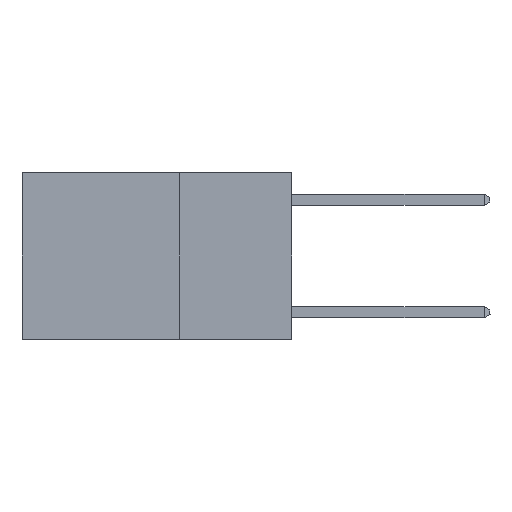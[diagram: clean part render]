
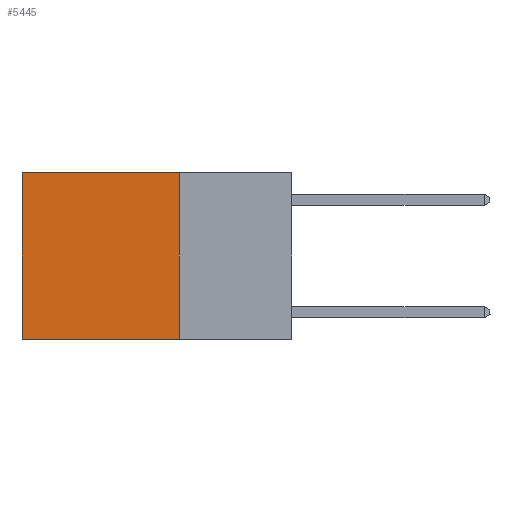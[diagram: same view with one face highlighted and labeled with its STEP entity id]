
A CAD part, left-side view. The second image highlights one B-rep face of the part: STEP entity #5445.
In plain terms, the highlighted planar face has unit normal (-1, 0, 0).
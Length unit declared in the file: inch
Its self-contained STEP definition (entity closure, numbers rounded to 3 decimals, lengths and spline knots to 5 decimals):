
#27 = CARTESIAN_POINT ( 'NONE',  ( 0.2625, 0.6, 0. ) ) ;
#120 = ORIENTED_EDGE ( 'NONE', *, *, #5655, .T. ) ;
#579 = CARTESIAN_POINT ( 'NONE',  ( 0.2625, 0.25, -0.37 ) ) ;
#905 = CARTESIAN_POINT ( 'NONE',  ( 0.2625, 0.6, 0. ) ) ;
#1513 = VECTOR ( 'NONE', #4620, 39.37008 ) ;
#1667 = CARTESIAN_POINT ( 'NONE',  ( 0.2625, 0.25, 0. ) ) ;
#3441 = VECTOR ( 'NONE', #10141, 39.37008 ) ;
#3451 = EDGE_CURVE ( 'NONE', #8773, #9184, #8191, .T. ) ;
#4213 = VERTEX_POINT ( 'NONE', #6761 ) ;
#4579 = EDGE_LOOP ( 'NONE', ( #120, #8152, #8358, #5119 ) ) ;
#4620 = DIRECTION ( 'NONE',  ( 0., 1., 0. ) ) ;
#4699 = AXIS2_PLACEMENT_3D ( 'NONE', #8420, #5802, #8320 ) ;
#4772 = CARTESIAN_POINT ( 'NONE',  ( 0.2625, 0.25, 0. ) ) ;
#4924 = EDGE_CURVE ( 'NONE', #5076, #4213, #8097, .T. ) ;
#5031 = DIRECTION ( 'NONE',  ( 0., 0., -1. ) ) ;
#5076 = VERTEX_POINT ( 'NONE', #579 ) ;
#5119 = ORIENTED_EDGE ( 'NONE', *, *, #3451, .T. ) ;
#5405 = VECTOR ( 'NONE', #5031, 39.37008 ) ;
#5445 = ADVANCED_FACE ( 'NONE', ( #9259 ), #11199, .F. ) ;
#5655 = EDGE_CURVE ( 'NONE', #9184, #4213, #6088, .T. ) ;
#5802 = DIRECTION ( 'NONE',  ( 1., 0., 0. ) ) ;
#5915 = LINE ( 'NONE', #9475, #5405 ) ;
#6088 = LINE ( 'NONE', #27, #7661 ) ;
#6350 = CARTESIAN_POINT ( 'NONE',  ( 0.2625, 0.25, -0.37 ) ) ;
#6761 = CARTESIAN_POINT ( 'NONE',  ( 0.2625, 0.6, -0.37 ) ) ;
#7661 = VECTOR ( 'NONE', #8988, 39.37008 ) ;
#8097 = LINE ( 'NONE', #6350, #1513 ) ;
#8152 = ORIENTED_EDGE ( 'NONE', *, *, #4924, .F. ) ;
#8191 = LINE ( 'NONE', #4772, #3441 ) ;
#8320 = DIRECTION ( 'NONE',  ( 0., 0., -1. ) ) ;
#8358 = ORIENTED_EDGE ( 'NONE', *, *, #10358, .F. ) ;
#8420 = CARTESIAN_POINT ( 'NONE',  ( 0.2625, 0.25, 0. ) ) ;
#8773 = VERTEX_POINT ( 'NONE', #1667 ) ;
#8988 = DIRECTION ( 'NONE',  ( 0., 0., -1. ) ) ;
#9184 = VERTEX_POINT ( 'NONE', #905 ) ;
#9259 = FACE_OUTER_BOUND ( 'NONE', #4579, .T. ) ;
#9475 = CARTESIAN_POINT ( 'NONE',  ( 0.2625, 0.25, 0. ) ) ;
#10141 = DIRECTION ( 'NONE',  ( 0., 1., 0. ) ) ;
#10358 = EDGE_CURVE ( 'NONE', #8773, #5076, #5915, .T. ) ;
#11199 = PLANE ( 'NONE',  #4699 ) ;
